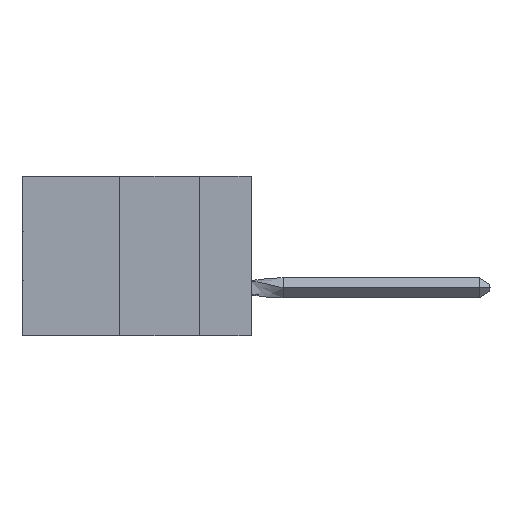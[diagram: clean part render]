
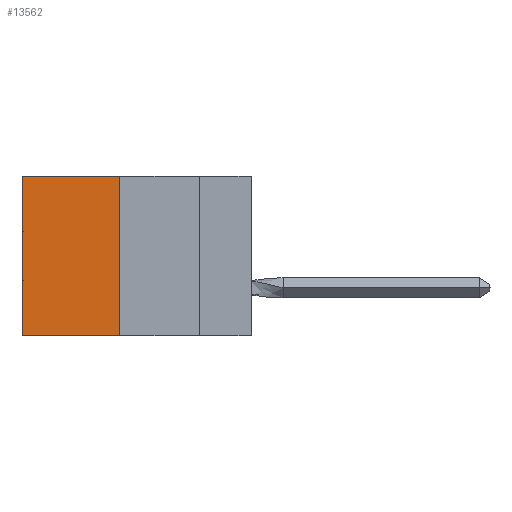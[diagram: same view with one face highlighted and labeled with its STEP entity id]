
A CAD part, left-side view. The second image highlights one B-rep face of the part: STEP entity #13562.
In plain terms, the highlighted planar face has unit normal (-1, 0, 0).
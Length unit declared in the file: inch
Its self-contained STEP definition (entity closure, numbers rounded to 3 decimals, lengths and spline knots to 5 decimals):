
#149 = LINE ( 'NONE', #25989, #29962 ) ;
#1823 = DIRECTION ( 'NONE',  ( 1., 0., 0. ) ) ;
#2664 = ORIENTED_EDGE ( 'NONE', *, *, #41054, .T. ) ;
#3575 = DIRECTION ( 'NONE',  ( 0., 0., -1. ) ) ;
#4387 = EDGE_CURVE ( 'NONE', #39105, #26212, #16416, .T. ) ;
#6679 = CARTESIAN_POINT ( 'NONE',  ( 0.305, 0.413, -0.5 ) ) ;
#6710 = VERTEX_POINT ( 'NONE', #25308 ) ;
#7410 = CARTESIAN_POINT ( 'NONE',  ( 0.305, 0.413, 0. ) ) ;
#9653 = CARTESIAN_POINT ( 'NONE',  ( 0.305, 0.413, -0.5 ) ) ;
#9913 = DIRECTION ( 'NONE',  ( 0., 1., 0. ) ) ;
#13069 = LINE ( 'NONE', #7410, #14133 ) ;
#13422 = EDGE_CURVE ( 'NONE', #26212, #25222, #149, .T. ) ;
#13562 = ADVANCED_FACE ( 'NONE', ( #25831 ), #30768, .F. ) ;
#14133 = VECTOR ( 'NONE', #35363, 39.37008 ) ;
#14866 = DIRECTION ( 'NONE',  ( 0., 0., -1. ) ) ;
#15088 = ORIENTED_EDGE ( 'NONE', *, *, #26265, .T. ) ;
#15365 = ORIENTED_EDGE ( 'NONE', *, *, #4387, .F. ) ;
#15803 = DIRECTION ( 'NONE',  ( 0., 0., -1. ) ) ;
#16416 = LINE ( 'NONE', #6679, #39089 ) ;
#21240 = VECTOR ( 'NONE', #15803, 39.37008 ) ;
#21952 = CARTESIAN_POINT ( 'NONE',  ( 0.305, 0.413, 0. ) ) ;
#25068 = ORIENTED_EDGE ( 'NONE', *, *, #13422, .F. ) ;
#25222 = VERTEX_POINT ( 'NONE', #32009 ) ;
#25308 = CARTESIAN_POINT ( 'NONE',  ( 0.305, 0.72, 0. ) ) ;
#25831 = FACE_OUTER_BOUND ( 'NONE', #29715, .T. ) ;
#25989 = CARTESIAN_POINT ( 'NONE',  ( 0.305, 0.413, -0.5 ) ) ;
#26212 = VERTEX_POINT ( 'NONE', #9653 ) ;
#26265 = EDGE_CURVE ( 'NONE', #39105, #6710, #13069, .T. ) ;
#29715 = EDGE_LOOP ( 'NONE', ( #2664, #25068, #15365, #15088 ) ) ;
#29962 = VECTOR ( 'NONE', #9913, 39.37008 ) ;
#30768 = PLANE ( 'NONE',  #31073 ) ;
#31073 = AXIS2_PLACEMENT_3D ( 'NONE', #34251, #1823, #14866 ) ;
#31970 = CARTESIAN_POINT ( 'NONE',  ( 0.305, 0.72, -0.5 ) ) ;
#32009 = CARTESIAN_POINT ( 'NONE',  ( 0.305, 0.72, -0.5 ) ) ;
#34251 = CARTESIAN_POINT ( 'NONE',  ( 0.305, 0.413, -0.5 ) ) ;
#35363 = DIRECTION ( 'NONE',  ( 0., 1., 0. ) ) ;
#39089 = VECTOR ( 'NONE', #3575, 39.37008 ) ;
#39105 = VERTEX_POINT ( 'NONE', #21952 ) ;
#41054 = EDGE_CURVE ( 'NONE', #6710, #25222, #41463, .T. ) ;
#41463 = LINE ( 'NONE', #31970, #21240 ) ;
